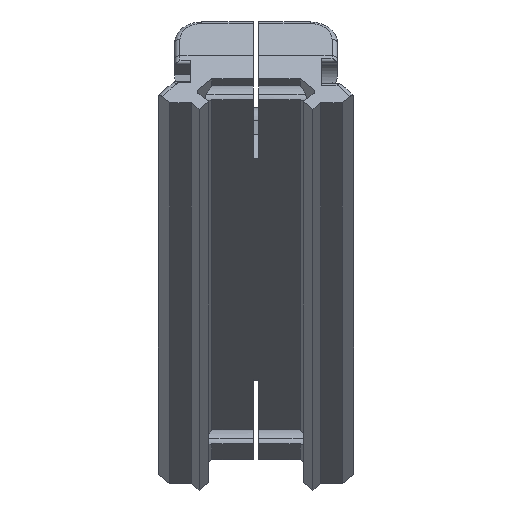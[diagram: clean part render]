
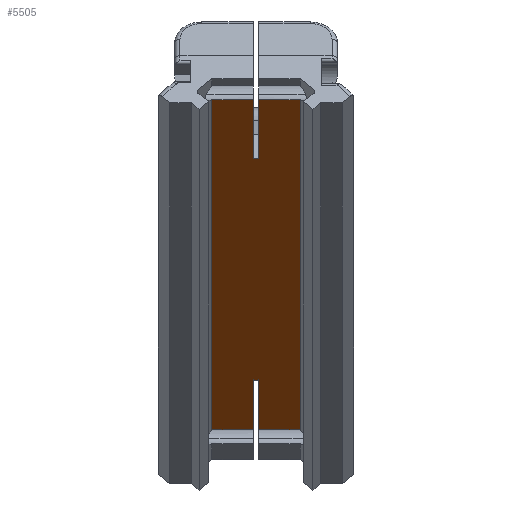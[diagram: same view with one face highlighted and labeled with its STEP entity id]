
A CAD part, top view. The second image highlights one B-rep face of the part: STEP entity #5505.
In plain terms, the highlighted planar face has unit normal (0, -0.819, 0.574).
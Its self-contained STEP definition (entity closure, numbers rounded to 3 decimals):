
#70 = ORIENTED_EDGE ( 'NONE', *, *, #11613, .F. ) ;
#472 = VECTOR ( 'NONE', #19495, 1000. ) ;
#617 = EDGE_CURVE ( 'NONE', #3244, #21206, #22214, .T. ) ;
#634 = CARTESIAN_POINT ( 'NONE',  ( -89.5, 0.723, 79.775 ) ) ;
#974 = CARTESIAN_POINT ( 'NONE',  ( -81.881, 11.45, 95.094 ) ) ;
#1014 = CARTESIAN_POINT ( 'NONE',  ( -90.5, 0.723, 79.775 ) ) ;
#1072 = LINE ( 'NONE', #17796, #14867 ) ;
#1099 = ORIENTED_EDGE ( 'NONE', *, *, #5182, .F. ) ;
#1249 = CARTESIAN_POINT ( 'NONE',  ( -81.881, -49.186, 8.497 ) ) ;
#1575 = CARTESIAN_POINT ( 'NONE',  ( -98.119, -82.79, -39.494 ) ) ;
#1687 = CARTESIAN_POINT ( 'NONE',  ( -105., -49.186, 8.497 ) ) ;
#1732 = LINE ( 'NONE', #14791, #10374 ) ;
#2007 = VECTOR ( 'NONE', #5898, 1000. ) ;
#2582 = CARTESIAN_POINT ( 'NONE',  ( -81.881, -82.79, -39.494 ) ) ;
#2652 = VECTOR ( 'NONE', #13759, 1000. ) ;
#2851 = FACE_OUTER_BOUND ( 'NONE', #16132, .T. ) ;
#3087 = CARTESIAN_POINT ( 'NONE',  ( -89.5, 15.292, 100.581 ) ) ;
#3218 = EDGE_CURVE ( 'NONE', #17309, #21206, #11840, .T. ) ;
#3244 = VERTEX_POINT ( 'NONE', #8639 ) ;
#4037 = ORIENTED_EDGE ( 'NONE', *, *, #3218, .T. ) ;
#4097 = CARTESIAN_POINT ( 'NONE',  ( -89.5, 0.723, 79.775 ) ) ;
#4171 = VERTEX_POINT ( 'NONE', #18523 ) ;
#4675 = VERTEX_POINT ( 'NONE', #4097 ) ;
#5182 = EDGE_CURVE ( 'NONE', #5290, #4675, #20965, .T. ) ;
#5290 = VERTEX_POINT ( 'NONE', #1014 ) ;
#5329 = CARTESIAN_POINT ( 'NONE',  ( -90.5, -49.186, 8.497 ) ) ;
#5483 = VERTEX_POINT ( 'NONE', #10293 ) ;
#5505 = ADVANCED_FACE ( 'NONE', ( #2851 ), #15587, .F. ) ;
#5698 = DIRECTION ( 'NONE',  ( 1., 0., 0. ) ) ;
#5898 = DIRECTION ( 'NONE',  ( 0., 0.574, 0.819 ) ) ;
#5985 = VECTOR ( 'NONE', #10015, 1000. ) ;
#6180 = DIRECTION ( 'NONE',  ( 0., -0.574, -0.819 ) ) ;
#6391 = ORIENTED_EDGE ( 'NONE', *, *, #9964, .T. ) ;
#6570 = ORIENTED_EDGE ( 'NONE', *, *, #15354, .F. ) ;
#6614 = LINE ( 'NONE', #2582, #2007 ) ;
#6913 = CARTESIAN_POINT ( 'NONE',  ( -90.5, -54.684, 0.645 ) ) ;
#7039 = ORIENTED_EDGE ( 'NONE', *, *, #22290, .T. ) ;
#7772 = VERTEX_POINT ( 'NONE', #17178 ) ;
#7949 = CARTESIAN_POINT ( 'NONE',  ( -89.5, -40.116, 21.451 ) ) ;
#8151 = VERTEX_POINT ( 'NONE', #7949 ) ;
#8414 = VECTOR ( 'NONE', #19027, 1000. ) ;
#8605 = ORIENTED_EDGE ( 'NONE', *, *, #17502, .F. ) ;
#8639 = CARTESIAN_POINT ( 'NONE',  ( -90.5, -40.116, 21.451 ) ) ;
#8719 = DIRECTION ( 'NONE',  ( 0., 0.819, -0.574 ) ) ;
#8886 = CARTESIAN_POINT ( 'NONE',  ( -98.119, -49.186, 8.497 ) ) ;
#8993 = VECTOR ( 'NONE', #16436, 1000. ) ;
#9783 = CARTESIAN_POINT ( 'NONE',  ( -89.5, -40.116, 21.451 ) ) ;
#9901 = VECTOR ( 'NONE', #16727, 1000. ) ;
#9964 = EDGE_CURVE ( 'NONE', #16013, #19156, #6614, .T. ) ;
#10015 = DIRECTION ( 'NONE',  ( 0., 0.574, 0.819 ) ) ;
#10293 = CARTESIAN_POINT ( 'NONE',  ( -90.5, 11.45, 95.094 ) ) ;
#10350 = EDGE_CURVE ( 'NONE', #5483, #5290, #1732, .T. ) ;
#10374 = VECTOR ( 'NONE', #6180, 1000. ) ;
#10559 = LINE ( 'NONE', #3087, #5985 ) ;
#10870 = VECTOR ( 'NONE', #11938, 1000. ) ;
#10923 = ORIENTED_EDGE ( 'NONE', *, *, #617, .F. ) ;
#11480 = CARTESIAN_POINT ( 'NONE',  ( -105., 11.45, 95.094 ) ) ;
#11613 = EDGE_CURVE ( 'NONE', #17309, #4171, #14952, .T. ) ;
#11840 = LINE ( 'NONE', #1687, #2652 ) ;
#11938 = DIRECTION ( 'NONE',  ( 0., 0.574, 0.819 ) ) ;
#12134 = CARTESIAN_POINT ( 'NONE',  ( -89.5, 11.45, 95.094 ) ) ;
#12718 = DIRECTION ( 'NONE',  ( 1., 0., 0. ) ) ;
#12933 = VECTOR ( 'NONE', #13326, 1000. ) ;
#13326 = DIRECTION ( 'NONE',  ( -1., 0., 0. ) ) ;
#13373 = ORIENTED_EDGE ( 'NONE', *, *, #18538, .T. ) ;
#13569 = LINE ( 'NONE', #14681, #8993 ) ;
#13759 = DIRECTION ( 'NONE',  ( 1., 0., 0. ) ) ;
#14263 = LINE ( 'NONE', #17757, #472 ) ;
#14491 = LINE ( 'NONE', #11480, #9901 ) ;
#14681 = CARTESIAN_POINT ( 'NONE',  ( -89.5, -54.684, 0.645 ) ) ;
#14791 = CARTESIAN_POINT ( 'NONE',  ( -90.5, 15.292, 100.581 ) ) ;
#14867 = VECTOR ( 'NONE', #5698, 1000. ) ;
#14922 = VERTEX_POINT ( 'NONE', #12134 ) ;
#14952 = LINE ( 'NONE', #1575, #10870 ) ;
#15270 = AXIS2_PLACEMENT_3D ( 'NONE', #19080, #8719, #20803 ) ;
#15354 = EDGE_CURVE ( 'NONE', #8151, #3244, #22153, .T. ) ;
#15587 = PLANE ( 'NONE',  #15270 ) ;
#16013 = VERTEX_POINT ( 'NONE', #1249 ) ;
#16132 = EDGE_LOOP ( 'NONE', ( #6570, #21579, #13373, #6391, #16296, #8605, #1099, #20066, #7039, #70, #4037, #10923 ) ) ;
#16296 = ORIENTED_EDGE ( 'NONE', *, *, #20792, .T. ) ;
#16394 = VECTOR ( 'NONE', #12718, 1000. ) ;
#16436 = DIRECTION ( 'NONE',  ( 0., 0.574, 0.819 ) ) ;
#16438 = EDGE_CURVE ( 'NONE', #7772, #8151, #13569, .T. ) ;
#16727 = DIRECTION ( 'NONE',  ( -1., 0., 0. ) ) ;
#17178 = CARTESIAN_POINT ( 'NONE',  ( -89.5, -49.186, 8.497 ) ) ;
#17309 = VERTEX_POINT ( 'NONE', #8886 ) ;
#17502 = EDGE_CURVE ( 'NONE', #4675, #14922, #10559, .T. ) ;
#17757 = CARTESIAN_POINT ( 'NONE',  ( -105., 11.45, 95.094 ) ) ;
#17796 = CARTESIAN_POINT ( 'NONE',  ( -105., -49.186, 8.497 ) ) ;
#18523 = CARTESIAN_POINT ( 'NONE',  ( -98.119, 11.45, 95.094 ) ) ;
#18538 = EDGE_CURVE ( 'NONE', #7772, #16013, #1072, .T. ) ;
#19027 = DIRECTION ( 'NONE',  ( 0., -0.574, -0.819 ) ) ;
#19080 = CARTESIAN_POINT ( 'NONE',  ( -98.119, -82.79, -39.494 ) ) ;
#19156 = VERTEX_POINT ( 'NONE', #974 ) ;
#19495 = DIRECTION ( 'NONE',  ( -1., 0., 0. ) ) ;
#20066 = ORIENTED_EDGE ( 'NONE', *, *, #10350, .F. ) ;
#20792 = EDGE_CURVE ( 'NONE', #19156, #14922, #14263, .T. ) ;
#20803 = DIRECTION ( 'NONE',  ( 1., 0., 0. ) ) ;
#20965 = LINE ( 'NONE', #634, #16394 ) ;
#21206 = VERTEX_POINT ( 'NONE', #5329 ) ;
#21579 = ORIENTED_EDGE ( 'NONE', *, *, #16438, .F. ) ;
#22153 = LINE ( 'NONE', #9783, #12933 ) ;
#22214 = LINE ( 'NONE', #6913, #8414 ) ;
#22290 = EDGE_CURVE ( 'NONE', #5483, #4171, #14491, .T. ) ;
